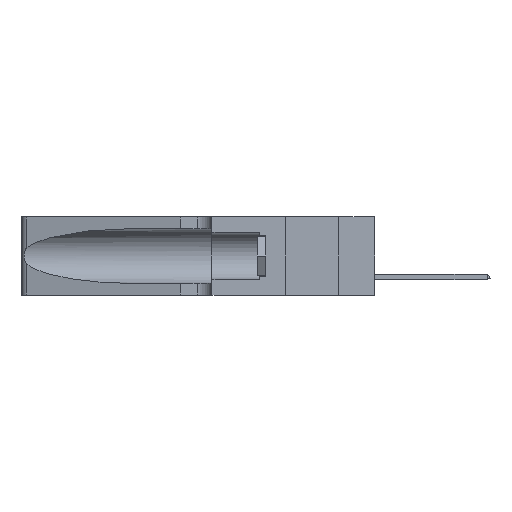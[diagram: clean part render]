
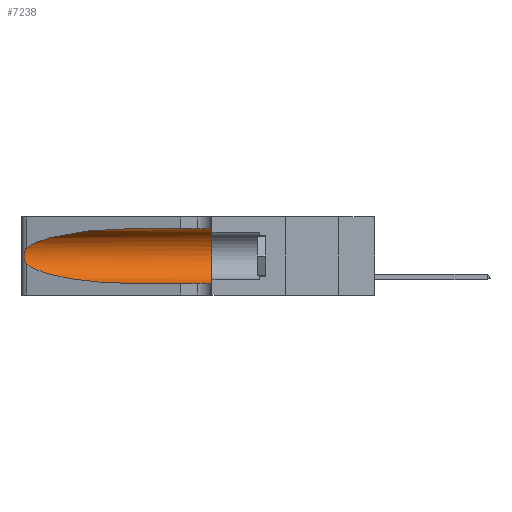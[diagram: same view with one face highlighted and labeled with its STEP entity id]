
A CAD part, left-side view. The second image highlights one B-rep face of the part: STEP entity #7238.
In plain terms, the highlighted cylindrical face has radius 3.308 mm (diameter 6.617 mm), a partial arc.
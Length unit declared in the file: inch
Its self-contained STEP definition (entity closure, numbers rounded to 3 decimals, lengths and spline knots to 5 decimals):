
#170 = EDGE_CURVE ( 'NONE', #14165, #14644, #21095, .T. ) ;
#1392 = CARTESIAN_POINT ( 'NONE',  ( 0.25854, 1.2359, 0.20912 ) ) ;
#1467 = CARTESIAN_POINT ( 'NONE',  ( 0.25639, 1.23184, 0.21858 ) ) ;
#1536 = CARTESIAN_POINT ( 'NONE',  ( 0.25787, 1.23484, 0.2124 ) ) ;
#2407 = VECTOR ( 'NONE', #17156, 39.37008 ) ;
#2493 = AXIS2_PLACEMENT_3D ( 'NONE', #21362, #6181, #6031 ) ;
#2618 = LINE ( 'NONE', #12130, #6765 ) ;
#2850 = CARTESIAN_POINT ( 'NONE',  ( 0.1305, 0.72297, 0.05475 ) ) ;
#2928 = ORIENTED_EDGE ( 'NONE', *, *, #16401, .T. ) ;
#3137 = CARTESIAN_POINT ( 'NONE',  ( 0.26017, 1.23833, 0.17102 ) ) ;
#3767 = CYLINDRICAL_SURFACE ( 'NONE', #16366, 0.13025 ) ;
#4504 = CARTESIAN_POINT ( 'NONE',  ( 0.25639, 1.23186, 0.15144 ) ) ;
#5326 = EDGE_CURVE ( 'NONE', #11396, #14495, #14292, .T. ) ;
#5373 = EDGE_CURVE ( 'NONE', #14644, #11396, #10398, .T. ) ;
#6031 = DIRECTION ( 'NONE',  ( 0., 0., 1. ) ) ;
#6085 = DIRECTION ( 'NONE',  ( 0., 0., -1. ) ) ;
#6181 = DIRECTION ( 'NONE',  ( 0., 1., 0. ) ) ;
#6765 = VECTOR ( 'NONE', #19044, 39.37008 ) ;
#6932 = CARTESIAN_POINT ( 'NONE',  ( 0.1305, 1.61858, 0.31525 ) ) ;
#7073 = ORIENTED_EDGE ( 'NONE', *, *, #170, .T. ) ;
#7238 = ADVANCED_FACE ( 'NONE', ( #21267 ), #3767, .F. ) ;
#7355 = CARTESIAN_POINT ( 'NONE',  ( 0.18966, 0.96281, 0.31525 ) ) ;
#7454 = VERTEX_POINT ( 'NONE', #10025 ) ;
#8143 = CARTESIAN_POINT ( 'NONE',  ( 0.25856, 1.23593, 0.16098 ) ) ;
#8364 = ORIENTED_EDGE ( 'NONE', *, *, #5373, .T. ) ;
#8608 = ORIENTED_EDGE ( 'NONE', *, *, #15376, .F. ) ;
#8622 = CARTESIAN_POINT ( 'NONE',  ( 0.1305, 0.72297, 0.31525 ) ) ;
#9062 = CARTESIAN_POINT ( 'NONE',  ( 0.2373, 1.15595, 0.28018 ) ) ;
#9085 = CARTESIAN_POINT ( 'NONE',  ( 0.25487, 1.22718, 0.14631 ) ) ;
#9132 = CARTESIAN_POINT ( 'NONE',  ( 0.25487, 1.22718, 0.22369 ) ) ;
#9448 = LINE ( 'NONE', #6932, #2407 ) ;
#9541 = CARTESIAN_POINT ( 'NONE',  ( 0.18966, 0.96281, 0.05475 ) ) ;
#10025 = CARTESIAN_POINT ( 'NONE',  ( 0.1305, 0.35, 0.31525 ) ) ;
#10398 = B_SPLINE_CURVE_WITH_KNOTS ( 'NONE', 3,
 ( #14739, #11449, #1467, #1536, #1392, #13059, #21440, #18137, #3137, #8143, #16340, #4504, #19821, #21291 ),
 .UNSPECIFIED., .F., .F.,
 ( 4, 2, 2, 2, 2, 2, 4 ),
 ( 0., 0.00027, 0.00053, 0.00107, 0.0016, 0.00187, 0.00214 ),
 .UNSPECIFIED. ) ;
#11396 = VERTEX_POINT ( 'NONE', #9085 ) ;
#11449 = CARTESIAN_POINT ( 'NONE',  ( 0.25555, 1.22994, 0.2215 ) ) ;
#12130 = CARTESIAN_POINT ( 'NONE',  ( 0.1305, 1.61858, 0.05475 ) ) ;
#12814 = CIRCLE ( 'NONE', #2493, 0.13025 ) ;
#13059 = CARTESIAN_POINT ( 'NONE',  ( 0.26018, 1.23835, 0.19895 ) ) ;
#14065 = EDGE_LOOP ( 'NONE', ( #7073, #8364, #18141, #2928, #8608, #21556 ) ) ;
#14165 = VERTEX_POINT ( 'NONE', #8622 ) ;
#14292 =( BOUNDED_CURVE ( )  B_SPLINE_CURVE ( 3, ( #14818, #19598, #9541, #2850 ),
 .UNSPECIFIED., .F., .T. ) 
 B_SPLINE_CURVE_WITH_KNOTS ( ( 4, 4 ),
 ( 3.44316, 4.71239 ),
 .UNSPECIFIED. ) 
 CURVE ( )  GEOMETRIC_REPRESENTATION_ITEM ( )  RATIONAL_B_SPLINE_CURVE ( ( 1., 0.87, 0.87, 1. ) ) 
 REPRESENTATION_ITEM ( '' )  );
#14428 = DIRECTION ( 'NONE',  ( 0., -1., 0. ) ) ;
#14495 = VERTEX_POINT ( 'NONE', #21227 ) ;
#14644 = VERTEX_POINT ( 'NONE', #19964 ) ;
#14739 = CARTESIAN_POINT ( 'NONE',  ( 0.25487, 1.22718, 0.22369 ) ) ;
#14818 = CARTESIAN_POINT ( 'NONE',  ( 0.25487, 1.22718, 0.14631 ) ) ;
#15376 = EDGE_CURVE ( 'NONE', #7454, #15881, #12814, .T. ) ;
#15881 = VERTEX_POINT ( 'NONE', #20604 ) ;
#16340 = CARTESIAN_POINT ( 'NONE',  ( 0.25789, 1.23486, 0.15765 ) ) ;
#16366 = AXIS2_PLACEMENT_3D ( 'NONE', #17766, #14428, #6085 ) ;
#16401 = EDGE_CURVE ( 'NONE', #14495, #15881, #2618, .T. ) ;
#17156 = DIRECTION ( 'NONE',  ( 0., -1., 0. ) ) ;
#17766 = CARTESIAN_POINT ( 'NONE',  ( 0.1305, 1.61858, 0.185 ) ) ;
#18137 = CARTESIAN_POINT ( 'NONE',  ( 0.26075, 1.23896, 0.178 ) ) ;
#18141 = ORIENTED_EDGE ( 'NONE', *, *, #5326, .T. ) ;
#19044 = DIRECTION ( 'NONE',  ( 0., -1., 0. ) ) ;
#19271 = CARTESIAN_POINT ( 'NONE',  ( 0.1305, 0.72297, 0.31525 ) ) ;
#19598 = CARTESIAN_POINT ( 'NONE',  ( 0.2373, 1.15595, 0.08982 ) ) ;
#19821 = CARTESIAN_POINT ( 'NONE',  ( 0.25555, 1.22993, 0.14849 ) ) ;
#19964 = CARTESIAN_POINT ( 'NONE',  ( 0.25487, 1.22718, 0.22369 ) ) ;
#20604 = CARTESIAN_POINT ( 'NONE',  ( 0.1305, 0.35, 0.05475 ) ) ;
#21095 =( BOUNDED_CURVE ( )  B_SPLINE_CURVE ( 3, ( #19271, #7355, #9062, #9132 ),
 .UNSPECIFIED., .F., .T. ) 
 B_SPLINE_CURVE_WITH_KNOTS ( ( 4, 4 ),
 ( 1.5708, 2.84003 ),
 .UNSPECIFIED. ) 
 CURVE ( )  GEOMETRIC_REPRESENTATION_ITEM ( )  RATIONAL_B_SPLINE_CURVE ( ( 1., 0.87, 0.87, 1. ) ) 
 REPRESENTATION_ITEM ( '' )  );
#21227 = CARTESIAN_POINT ( 'NONE',  ( 0.1305, 0.72297, 0.05475 ) ) ;
#21267 = FACE_OUTER_BOUND ( 'NONE', #14065, .T. ) ;
#21291 = CARTESIAN_POINT ( 'NONE',  ( 0.25487, 1.22718, 0.14631 ) ) ;
#21362 = CARTESIAN_POINT ( 'NONE',  ( 0.1305, 0.35, 0.185 ) ) ;
#21399 = EDGE_CURVE ( 'NONE', #14165, #7454, #9448, .T. ) ;
#21440 = CARTESIAN_POINT ( 'NONE',  ( 0.26075, 1.23896, 0.19203 ) ) ;
#21556 = ORIENTED_EDGE ( 'NONE', *, *, #21399, .F. ) ;
